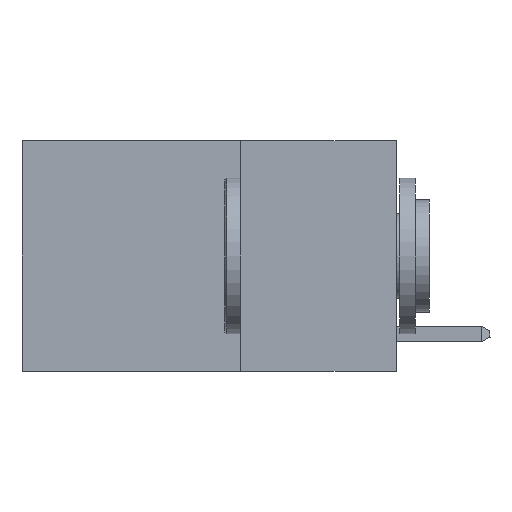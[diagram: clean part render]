
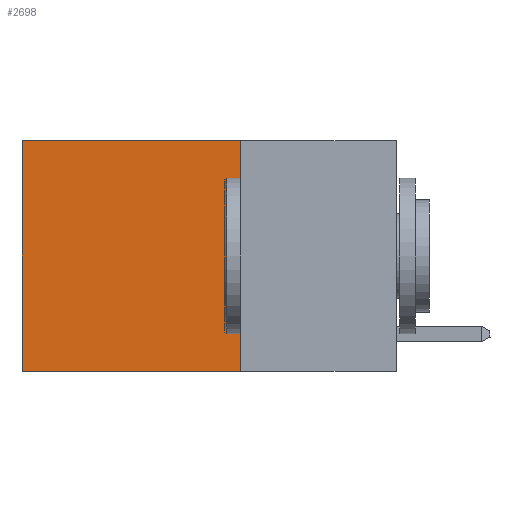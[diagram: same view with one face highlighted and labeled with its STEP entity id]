
A CAD part, left-side view. The second image highlights one B-rep face of the part: STEP entity #2698.
In plain terms, the highlighted planar face has unit normal (-1, 0, 0).
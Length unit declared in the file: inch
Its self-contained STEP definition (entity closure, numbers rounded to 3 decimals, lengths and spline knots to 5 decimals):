
#586 = EDGE_CURVE ( 'NONE', #6481, #3153, #3040, .T. ) ;
#710 = FACE_OUTER_BOUND ( 'NONE', #3121, .T. ) ;
#1136 = ORIENTED_EDGE ( 'NONE', *, *, #8743, .F. ) ;
#1531 = CARTESIAN_POINT ( 'NONE',  ( 0.2625, 0.25, 0. ) ) ;
#1609 = LINE ( 'NONE', #3401, #5714 ) ;
#1633 = EDGE_CURVE ( 'NONE', #6027, #7997, #1609, .T. ) ;
#2162 = CARTESIAN_POINT ( 'NONE',  ( 0.2625, 0.6, 0. ) ) ;
#2212 = DIRECTION ( 'NONE',  ( 0., 0., -1. ) ) ;
#2248 = DIRECTION ( 'NONE',  ( 1., 0., 0. ) ) ;
#2307 = PLANE ( 'NONE',  #6273 ) ;
#2477 = CARTESIAN_POINT ( 'NONE',  ( 0.2625, 0.25, 0. ) ) ;
#2698 = ADVANCED_FACE ( 'NONE', ( #710 ), #2307, .F. ) ;
#3040 = LINE ( 'NONE', #7943, #9045 ) ;
#3121 = EDGE_LOOP ( 'NONE', ( #4098, #1136, #9210, #5288 ) ) ;
#3153 = VERTEX_POINT ( 'NONE', #7635 ) ;
#3401 = CARTESIAN_POINT ( 'NONE',  ( 0.2625, 0.6, 0. ) ) ;
#4098 = ORIENTED_EDGE ( 'NONE', *, *, #1633, .T. ) ;
#4853 = VECTOR ( 'NONE', #8842, 39.37008 ) ;
#5084 = LINE ( 'NONE', #9611, #4853 ) ;
#5288 = ORIENTED_EDGE ( 'NONE', *, *, #5381, .T. ) ;
#5381 = EDGE_CURVE ( 'NONE', #6481, #6027, #8360, .T. ) ;
#5714 = VECTOR ( 'NONE', #7016, 39.37008 ) ;
#6027 = VERTEX_POINT ( 'NONE', #2162 ) ;
#6273 = AXIS2_PLACEMENT_3D ( 'NONE', #2477, #2248, #2212 ) ;
#6339 = VECTOR ( 'NONE', #7925, 39.37008 ) ;
#6481 = VERTEX_POINT ( 'NONE', #7416 ) ;
#7016 = DIRECTION ( 'NONE',  ( 0., 0., -1. ) ) ;
#7416 = CARTESIAN_POINT ( 'NONE',  ( 0.2625, 0.25, 0. ) ) ;
#7635 = CARTESIAN_POINT ( 'NONE',  ( 0.2625, 0.25, -0.37 ) ) ;
#7913 = DIRECTION ( 'NONE',  ( 0., 0., -1. ) ) ;
#7925 = DIRECTION ( 'NONE',  ( 0., 1., 0. ) ) ;
#7943 = CARTESIAN_POINT ( 'NONE',  ( 0.2625, 0.25, 0. ) ) ;
#7997 = VERTEX_POINT ( 'NONE', #8917 ) ;
#8360 = LINE ( 'NONE', #1531, #6339 ) ;
#8743 = EDGE_CURVE ( 'NONE', #3153, #7997, #5084, .T. ) ;
#8842 = DIRECTION ( 'NONE',  ( 0., 1., 0. ) ) ;
#8917 = CARTESIAN_POINT ( 'NONE',  ( 0.2625, 0.6, -0.37 ) ) ;
#9045 = VECTOR ( 'NONE', #7913, 39.37008 ) ;
#9210 = ORIENTED_EDGE ( 'NONE', *, *, #586, .F. ) ;
#9611 = CARTESIAN_POINT ( 'NONE',  ( 0.2625, 0.25, -0.37 ) ) ;
